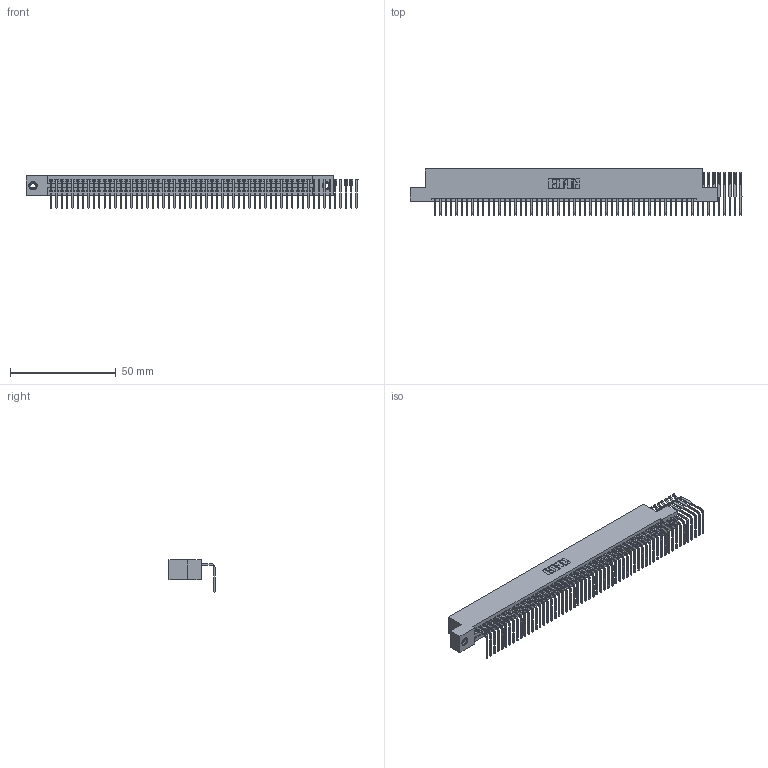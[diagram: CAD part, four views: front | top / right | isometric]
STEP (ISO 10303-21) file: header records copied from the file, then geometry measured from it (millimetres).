
FILE_DESCRIPTION (( 'STEP AP203' ), '1' );
FILE_NAME ('345-058-558-108.STEP', '2019-10-10T20:06:31', ( '' ), ( '' ), 'SwSTEP 2.0', 'SolidWorks 2016', '' );
FILE_SCHEMA (( 'CONFIG_CONTROL_DESIGN' ));
Length unit declared in the file: inch
Products named in the file (4): 345-250-001_345-250-003-102; 345-058-558-108; 345 Part_Flush Mounting Lugs - 0.156 Dia-TI; 345-292-001_558 Tail - 2
Assembly tree (61 placements, depth 2):
  345-058-558-108
    345 Part_Flush Mounting Lugs - 0.156 Dia-TI
    345-292-001_558 Tail - 2  x58
    345-250-001_345-250-003-102  x2
Bounding box: 157.29 x 21.83 x 15.37 mm (x, y, z)
Volume: 14182.9 mm3; surface area: 20644.9 mm2
Topology: 61 solids, 61 shells, 3522 faces, 10547 edges, 6946 vertices
Faces by surface type: plane 2422, cylinder 1084, cone 12, torus 4
Entity records: 37494 total; most frequent: CARTESIAN_POINT 6435, ORIENTED_EDGE 6402, DIRECTION 5647, EDGE_CURVE 3201, LINE 2853, VECTOR 2853, VERTEX_POINT 2128, AXIS2_PLACEMENT_3D 1397
